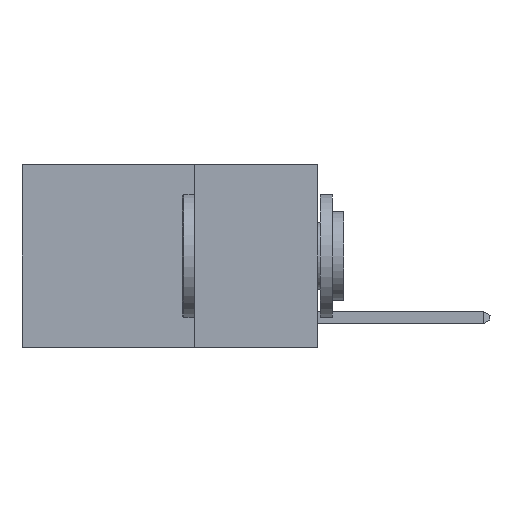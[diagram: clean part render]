
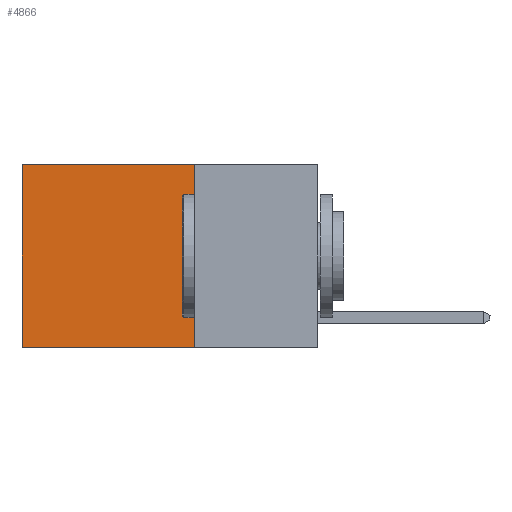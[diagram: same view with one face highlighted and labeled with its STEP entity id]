
A CAD part, left-side view. The second image highlights one B-rep face of the part: STEP entity #4866.
In plain terms, the highlighted planar face has unit normal (-1, 0, 0).
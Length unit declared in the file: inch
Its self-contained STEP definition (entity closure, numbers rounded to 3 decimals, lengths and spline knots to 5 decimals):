
#26 = LINE ( 'NONE', #8530, #354 ) ;
#142 = ORIENTED_EDGE ( 'NONE', *, *, #5450, .T. ) ;
#168 = ORIENTED_EDGE ( 'NONE', *, *, #3871, .F. ) ;
#283 = CARTESIAN_POINT ( 'NONE',  ( 0.2625, 0.25, 0. ) ) ;
#354 = VECTOR ( 'NONE', #2873, 39.37008 ) ;
#373 = CARTESIAN_POINT ( 'NONE',  ( 0.2625, 0.6, 0. ) ) ;
#410 = ORIENTED_EDGE ( 'NONE', *, *, #6659, .F. ) ;
#571 = CARTESIAN_POINT ( 'NONE',  ( 0.2625, 0.25, -0.37 ) ) ;
#588 = ORIENTED_EDGE ( 'NONE', *, *, #5201, .T. ) ;
#869 = PLANE ( 'NONE',  #11068 ) ;
#1709 = VERTEX_POINT ( 'NONE', #1873 ) ;
#1840 = DIRECTION ( 'NONE',  ( 1., 0., 0. ) ) ;
#1873 = CARTESIAN_POINT ( 'NONE',  ( 0.2625, 0.25, -0.37 ) ) ;
#2873 = DIRECTION ( 'NONE',  ( 0., 0., -1. ) ) ;
#3011 = CARTESIAN_POINT ( 'NONE',  ( 0.2625, 0.25, 0. ) ) ;
#3291 = FACE_OUTER_BOUND ( 'NONE', #11350, .T. ) ;
#3588 = VECTOR ( 'NONE', #5404, 39.37008 ) ;
#3871 = EDGE_CURVE ( 'NONE', #1709, #6035, #8313, .T. ) ;
#4463 = VERTEX_POINT ( 'NONE', #373 ) ;
#4833 = CARTESIAN_POINT ( 'NONE',  ( 0.2625, 0.25, 0. ) ) ;
#4866 = ADVANCED_FACE ( 'NONE', ( #3291 ), #869, .F. ) ;
#5201 = EDGE_CURVE ( 'NONE', #7293, #4463, #7756, .T. ) ;
#5404 = DIRECTION ( 'NONE',  ( 0., 1., 0. ) ) ;
#5450 = EDGE_CURVE ( 'NONE', #4463, #6035, #26, .T. ) ;
#6035 = VERTEX_POINT ( 'NONE', #6124 ) ;
#6105 = DIRECTION ( 'NONE',  ( 0., 1., 0. ) ) ;
#6124 = CARTESIAN_POINT ( 'NONE',  ( 0.2625, 0.6, -0.37 ) ) ;
#6659 = EDGE_CURVE ( 'NONE', #7293, #1709, #8573, .T. ) ;
#7293 = VERTEX_POINT ( 'NONE', #4833 ) ;
#7756 = LINE ( 'NONE', #283, #10147 ) ;
#8269 = VECTOR ( 'NONE', #9577, 39.37008 ) ;
#8313 = LINE ( 'NONE', #571, #3588 ) ;
#8456 = CARTESIAN_POINT ( 'NONE',  ( 0.2625, 0.25, 0. ) ) ;
#8499 = DIRECTION ( 'NONE',  ( 0., 0., -1. ) ) ;
#8530 = CARTESIAN_POINT ( 'NONE',  ( 0.2625, 0.6, 0. ) ) ;
#8573 = LINE ( 'NONE', #3011, #8269 ) ;
#9577 = DIRECTION ( 'NONE',  ( 0., 0., -1. ) ) ;
#10147 = VECTOR ( 'NONE', #6105, 39.37008 ) ;
#11068 = AXIS2_PLACEMENT_3D ( 'NONE', #8456, #1840, #8499 ) ;
#11350 = EDGE_LOOP ( 'NONE', ( #142, #168, #410, #588 ) ) ;
